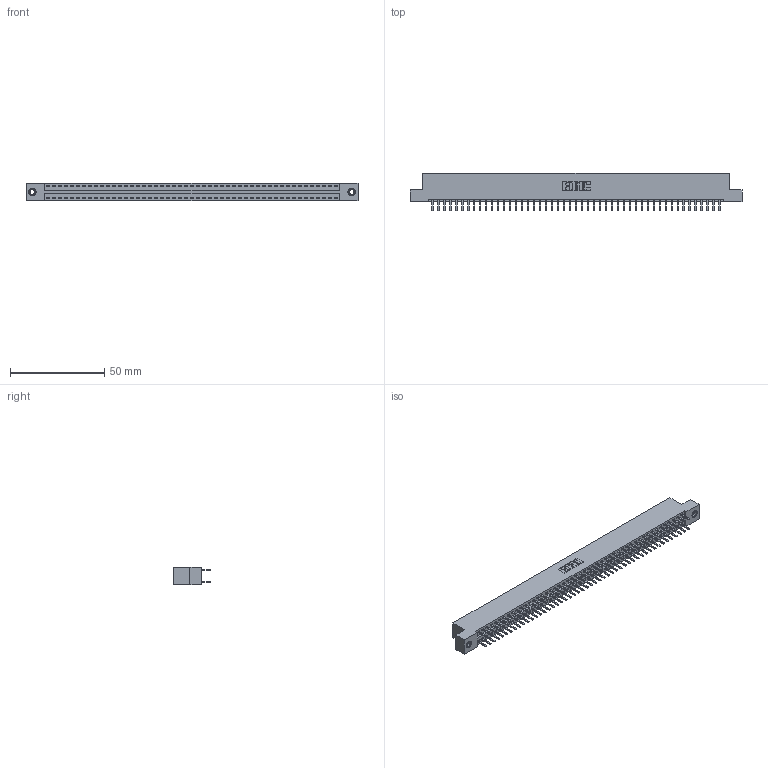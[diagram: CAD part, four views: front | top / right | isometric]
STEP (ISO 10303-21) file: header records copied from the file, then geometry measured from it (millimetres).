
FILE_DESCRIPTION (( 'STEP AP203' ), '1' );
FILE_NAME ('346-098-520-207.STEP', '2022-05-26T17:41:01', ( '' ), ( '' ), 'SwSTEP 2.0', 'SolidWorks 2020', '' );
FILE_SCHEMA (( 'CONFIG_CONTROL_DESIGN' ));
Length unit declared in the file: inch
Products named in the file (4): 346-098-520-207; 345-250-001_345-250-005-103; 345-292-001_345-293-120; 346 Part_Flush Mounting Lugs - 0.156 Dia-TI
Assembly tree (101 placements, depth 2):
  346-098-520-207
    346 Part_Flush Mounting Lugs - 0.156 Dia-TI
    345-292-001_345-293-120  x98
    345-250-001_345-250-005-103  x2
Bounding box: 176.15 x 20.02 x 9.4 mm (x, y, z)
Volume: 17174.5 mm3; surface area: 23650.3 mm2
Topology: 101 solids, 101 shells, 5670 faces, 16439 edges, 10690 vertices
Faces by surface type: plane 3734, cylinder 1920, cone 12, torus 4
Entity records: 32336 total; most frequent: CARTESIAN_POINT 5315, ORIENTED_EDGE 5230, DIRECTION 4749, EDGE_CURVE 2615, VECTOR 2263, LINE 2263, VERTEX_POINT 1736, AXIS2_PLACEMENT_3D 1243
